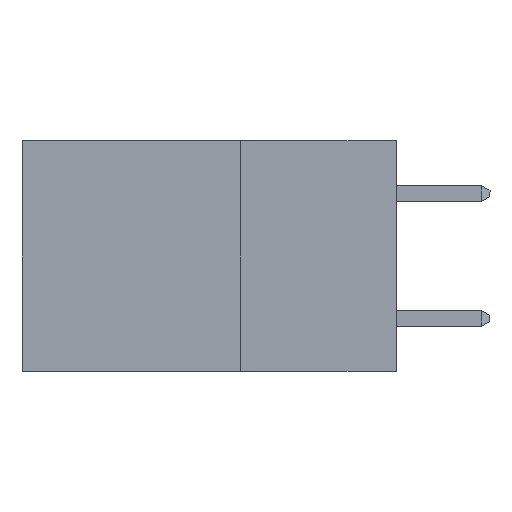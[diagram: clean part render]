
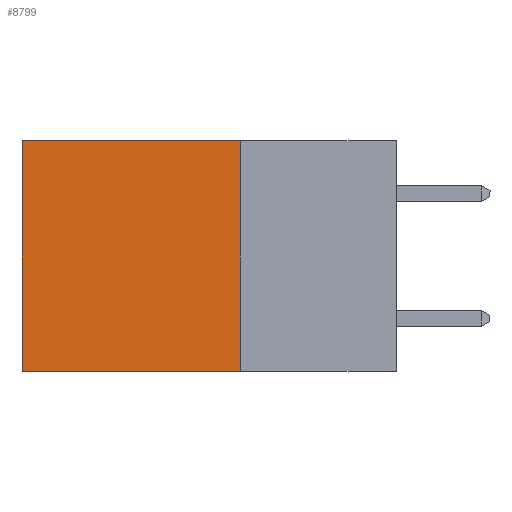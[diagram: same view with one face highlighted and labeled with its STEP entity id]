
A CAD part, left-side view. The second image highlights one B-rep face of the part: STEP entity #8799.
In plain terms, the highlighted planar face has unit normal (-1, 0, 0).
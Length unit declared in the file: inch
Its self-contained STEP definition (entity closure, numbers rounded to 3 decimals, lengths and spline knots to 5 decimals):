
#126 = CARTESIAN_POINT ( 'NONE',  ( 0.2615, 0.25, -0.37 ) ) ;
#302 = CARTESIAN_POINT ( 'NONE',  ( 0.2615, 0.25, -0.37 ) ) ;
#942 = LINE ( 'NONE', #6941, #1806 ) ;
#1010 = AXIS2_PLACEMENT_3D ( 'NONE', #302, #5308, #6633 ) ;
#1043 = VECTOR ( 'NONE', #7637, 39.37008 ) ;
#1447 = VERTEX_POINT ( 'NONE', #8801 ) ;
#1651 = CARTESIAN_POINT ( 'NONE',  ( 0.2615, 0.25, -0.37 ) ) ;
#1806 = VECTOR ( 'NONE', #1891, 39.37008 ) ;
#1891 = DIRECTION ( 'NONE',  ( 0., 0., -1. ) ) ;
#2156 = CARTESIAN_POINT ( 'NONE',  ( 0.2615, 0.25, 0. ) ) ;
#2247 = DIRECTION ( 'NONE',  ( 0., 0., -1. ) ) ;
#3090 = CARTESIAN_POINT ( 'NONE',  ( 0.2615, 0.6, 0. ) ) ;
#3596 = EDGE_LOOP ( 'NONE', ( #5661, #3824, #9265, #8835 ) ) ;
#3824 = ORIENTED_EDGE ( 'NONE', *, *, #4557, .F. ) ;
#4449 = VERTEX_POINT ( 'NONE', #126 ) ;
#4557 = EDGE_CURVE ( 'NONE', #4449, #1447, #8382, .T. ) ;
#4912 = VERTEX_POINT ( 'NONE', #6600 ) ;
#5122 = LINE ( 'NONE', #5171, #9357 ) ;
#5171 = CARTESIAN_POINT ( 'NONE',  ( 0.2615, 0.25, -0.37 ) ) ;
#5308 = DIRECTION ( 'NONE',  ( 1., 0., 0. ) ) ;
#5661 = ORIENTED_EDGE ( 'NONE', *, *, #8025, .T. ) ;
#6600 = CARTESIAN_POINT ( 'NONE',  ( 0.2615, 0.25, 0. ) ) ;
#6633 = DIRECTION ( 'NONE',  ( 0., 0., -1. ) ) ;
#6941 = CARTESIAN_POINT ( 'NONE',  ( 0.2615, 0.6, -0.37 ) ) ;
#7001 = FACE_OUTER_BOUND ( 'NONE', #3596, .T. ) ;
#7052 = PLANE ( 'NONE',  #1010 ) ;
#7637 = DIRECTION ( 'NONE',  ( 0., 1., 0. ) ) ;
#8025 = EDGE_CURVE ( 'NONE', #8184, #1447, #942, .T. ) ;
#8100 = DIRECTION ( 'NONE',  ( 0., 1., 0. ) ) ;
#8184 = VERTEX_POINT ( 'NONE', #3090 ) ;
#8382 = LINE ( 'NONE', #1651, #1043 ) ;
#8748 = LINE ( 'NONE', #2156, #9193 ) ;
#8799 = ADVANCED_FACE ( 'NONE', ( #7001 ), #7052, .F. ) ;
#8801 = CARTESIAN_POINT ( 'NONE',  ( 0.2615, 0.6, -0.37 ) ) ;
#8835 = ORIENTED_EDGE ( 'NONE', *, *, #9263, .T. ) ;
#8880 = EDGE_CURVE ( 'NONE', #4912, #4449, #5122, .T. ) ;
#9193 = VECTOR ( 'NONE', #8100, 39.37008 ) ;
#9263 = EDGE_CURVE ( 'NONE', #4912, #8184, #8748, .T. ) ;
#9265 = ORIENTED_EDGE ( 'NONE', *, *, #8880, .F. ) ;
#9357 = VECTOR ( 'NONE', #2247, 39.37008 ) ;
